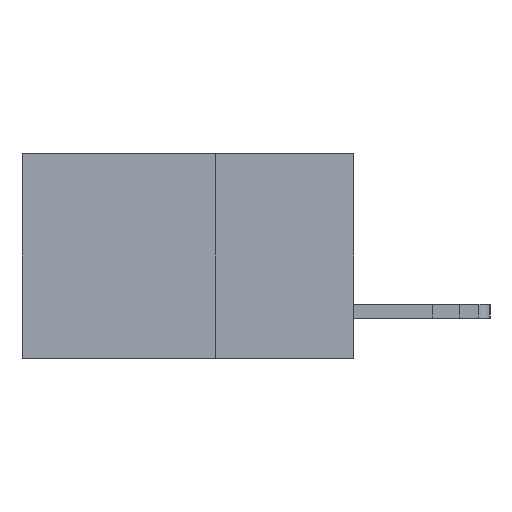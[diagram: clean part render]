
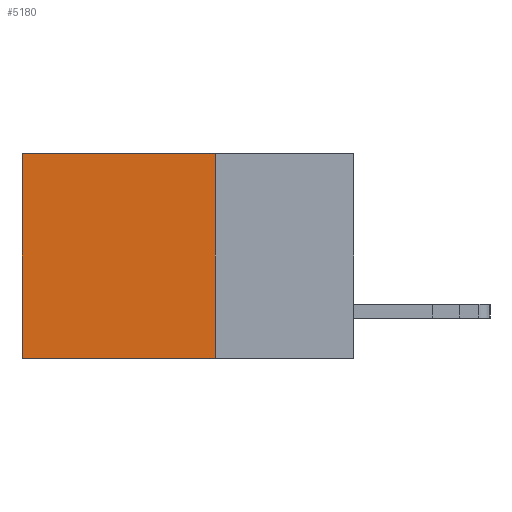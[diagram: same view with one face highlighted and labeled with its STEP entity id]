
A CAD part, left-side view. The second image highlights one B-rep face of the part: STEP entity #5180.
In plain terms, the highlighted planar face has unit normal (-1, 0, 0).
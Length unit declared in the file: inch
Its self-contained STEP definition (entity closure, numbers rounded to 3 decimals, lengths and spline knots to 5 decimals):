
#34 = CARTESIAN_POINT ( 'NONE',  ( 0.2875, 0.25, -0.37 ) ) ;
#889 = EDGE_CURVE ( 'NONE', #10527, #12826, #1143, .T. ) ;
#1143 = LINE ( 'NONE', #6683, #15357 ) ;
#1289 = EDGE_LOOP ( 'NONE', ( #6420, #7823, #12748, #2743 ) ) ;
#1407 = DIRECTION ( 'NONE',  ( 0., 1., 0. ) ) ;
#2122 = AXIS2_PLACEMENT_3D ( 'NONE', #16152, #3816, #13255 ) ;
#2743 = ORIENTED_EDGE ( 'NONE', *, *, #8290, .T. ) ;
#2778 = VERTEX_POINT ( 'NONE', #5977 ) ;
#3262 = CARTESIAN_POINT ( 'NONE',  ( 0.2875, 0.6, 0. ) ) ;
#3816 = DIRECTION ( 'NONE',  ( 1., 0., 0. ) ) ;
#4006 = LINE ( 'NONE', #9521, #14401 ) ;
#5180 = ADVANCED_FACE ( 'NONE', ( #7670 ), #16250, .F. ) ;
#5977 = CARTESIAN_POINT ( 'NONE',  ( 0.2875, 0.6, -0.37 ) ) ;
#6420 = ORIENTED_EDGE ( 'NONE', *, *, #7616, .T. ) ;
#6457 = CARTESIAN_POINT ( 'NONE',  ( 0.2875, 0.25, 0. ) ) ;
#6570 = VECTOR ( 'NONE', #12008, 39.37008 ) ;
#6683 = CARTESIAN_POINT ( 'NONE',  ( 0.2875, 0.25, 0. ) ) ;
#7616 = EDGE_CURVE ( 'NONE', #10659, #2778, #4006, .T. ) ;
#7670 = FACE_OUTER_BOUND ( 'NONE', #1289, .T. ) ;
#7823 = ORIENTED_EDGE ( 'NONE', *, *, #11434, .F. ) ;
#8290 = EDGE_CURVE ( 'NONE', #10527, #10659, #17545, .T. ) ;
#8666 = VECTOR ( 'NONE', #1407, 39.37008 ) ;
#9431 = DIRECTION ( 'NONE',  ( 0., 0., -1. ) ) ;
#9521 = CARTESIAN_POINT ( 'NONE',  ( 0.2875, 0.6, 0. ) ) ;
#9660 = LINE ( 'NONE', #16922, #8666 ) ;
#10527 = VERTEX_POINT ( 'NONE', #10735 ) ;
#10659 = VERTEX_POINT ( 'NONE', #3262 ) ;
#10735 = CARTESIAN_POINT ( 'NONE',  ( 0.2875, 0.25, 0. ) ) ;
#11434 = EDGE_CURVE ( 'NONE', #12826, #2778, #9660, .T. ) ;
#12008 = DIRECTION ( 'NONE',  ( 0., 1., 0. ) ) ;
#12246 = DIRECTION ( 'NONE',  ( 0., 0., -1. ) ) ;
#12748 = ORIENTED_EDGE ( 'NONE', *, *, #889, .F. ) ;
#12826 = VERTEX_POINT ( 'NONE', #34 ) ;
#13255 = DIRECTION ( 'NONE',  ( 0., 0., -1. ) ) ;
#14401 = VECTOR ( 'NONE', #9431, 39.37008 ) ;
#15357 = VECTOR ( 'NONE', #12246, 39.37008 ) ;
#16152 = CARTESIAN_POINT ( 'NONE',  ( 0.2875, 0.25, 0. ) ) ;
#16250 = PLANE ( 'NONE',  #2122 ) ;
#16922 = CARTESIAN_POINT ( 'NONE',  ( 0.2875, 0.25, -0.37 ) ) ;
#17545 = LINE ( 'NONE', #6457, #6570 ) ;
